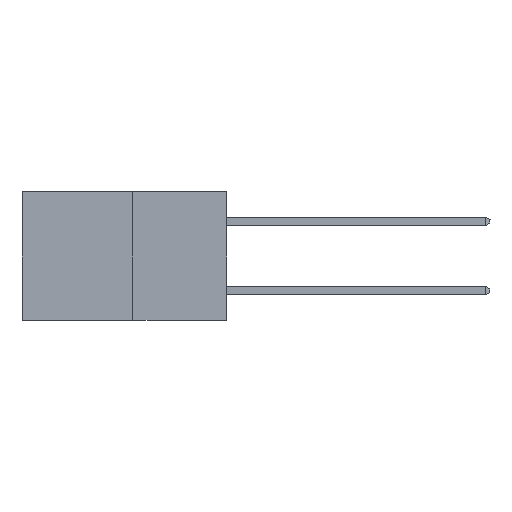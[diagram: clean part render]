
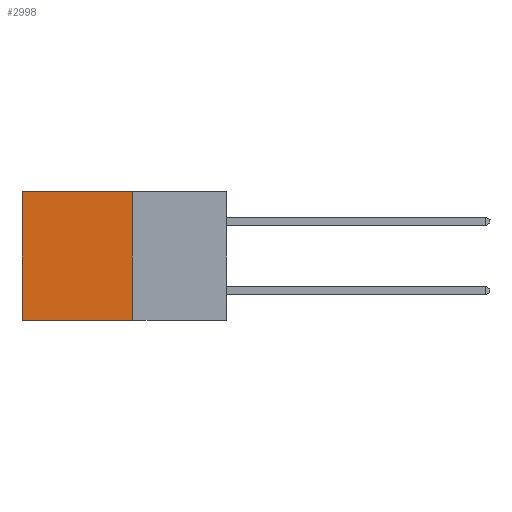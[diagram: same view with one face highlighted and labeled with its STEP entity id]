
A CAD part, left-side view. The second image highlights one B-rep face of the part: STEP entity #2998.
In plain terms, the highlighted planar face has unit normal (-1, 0, 0).
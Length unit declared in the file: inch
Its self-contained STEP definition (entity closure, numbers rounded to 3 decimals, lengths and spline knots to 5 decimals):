
#344 = DIRECTION ( 'NONE',  ( 0., 0., -1. ) ) ;
#1675 = ORIENTED_EDGE ( 'NONE', *, *, #6352, .F. ) ;
#2998 = ADVANCED_FACE ( 'NONE', ( #33048 ), #13985, .F. ) ;
#3720 = DIRECTION ( 'NONE',  ( 0., 1., 0. ) ) ;
#4577 = EDGE_CURVE ( 'NONE', #4604, #15185, #26140, .T. ) ;
#4604 = VERTEX_POINT ( 'NONE', #32757 ) ;
#5490 = CARTESIAN_POINT ( 'NONE',  ( 0.277, 0.59, 0. ) ) ;
#6352 = EDGE_CURVE ( 'NONE', #10149, #4604, #32992, .T. ) ;
#7573 = EDGE_CURVE ( 'NONE', #10149, #12729, #15134, .T. ) ;
#8084 = VECTOR ( 'NONE', #20832, 39.37008 ) ;
#9448 = CARTESIAN_POINT ( 'NONE',  ( 0.277, 0.59, -0.37 ) ) ;
#10149 = VERTEX_POINT ( 'NONE', #19913 ) ;
#10194 = ORIENTED_EDGE ( 'NONE', *, *, #14983, .T. ) ;
#12729 = VERTEX_POINT ( 'NONE', #5490 ) ;
#13759 = DIRECTION ( 'NONE',  ( 0., 0., -1. ) ) ;
#13872 = DIRECTION ( 'NONE',  ( 1., 0., 0. ) ) ;
#13985 = PLANE ( 'NONE',  #23372 ) ;
#14593 = CARTESIAN_POINT ( 'NONE',  ( 0.277, 0.27, -0.37 ) ) ;
#14983 = EDGE_CURVE ( 'NONE', #12729, #15185, #26390, .T. ) ;
#15134 = LINE ( 'NONE', #18168, #8084 ) ;
#15185 = VERTEX_POINT ( 'NONE', #28768 ) ;
#16001 = ORIENTED_EDGE ( 'NONE', *, *, #4577, .F. ) ;
#18168 = CARTESIAN_POINT ( 'NONE',  ( 0.277, 0.27, 0. ) ) ;
#19593 = CARTESIAN_POINT ( 'NONE',  ( 0.277, 0.27, -0.37 ) ) ;
#19913 = CARTESIAN_POINT ( 'NONE',  ( 0.277, 0.27, 0. ) ) ;
#20167 = VECTOR ( 'NONE', #27955, 39.37008 ) ;
#20832 = DIRECTION ( 'NONE',  ( 0., 1., 0. ) ) ;
#22474 = EDGE_LOOP ( 'NONE', ( #10194, #16001, #1675, #25142 ) ) ;
#23372 = AXIS2_PLACEMENT_3D ( 'NONE', #14593, #13872, #13759 ) ;
#25142 = ORIENTED_EDGE ( 'NONE', *, *, #7573, .T. ) ;
#25165 = VECTOR ( 'NONE', #344, 39.37008 ) ;
#26140 = LINE ( 'NONE', #19593, #31472 ) ;
#26390 = LINE ( 'NONE', #9448, #20167 ) ;
#27955 = DIRECTION ( 'NONE',  ( 0., 0., -1. ) ) ;
#28768 = CARTESIAN_POINT ( 'NONE',  ( 0.277, 0.59, -0.37 ) ) ;
#31472 = VECTOR ( 'NONE', #3720, 39.37008 ) ;
#32073 = CARTESIAN_POINT ( 'NONE',  ( 0.277, 0.27, -0.37 ) ) ;
#32757 = CARTESIAN_POINT ( 'NONE',  ( 0.277, 0.27, -0.37 ) ) ;
#32992 = LINE ( 'NONE', #32073, #25165 ) ;
#33048 = FACE_OUTER_BOUND ( 'NONE', #22474, .T. ) ;
